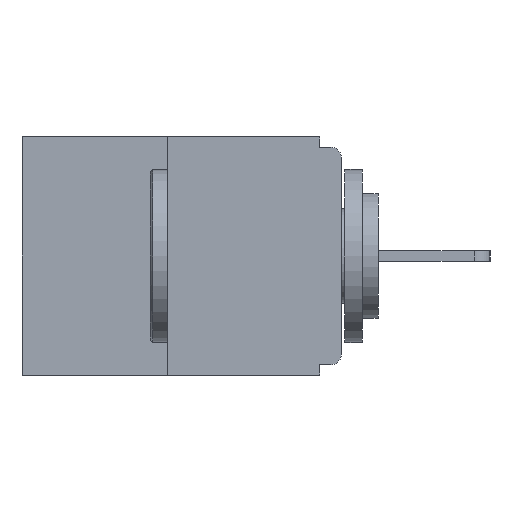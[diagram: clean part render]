
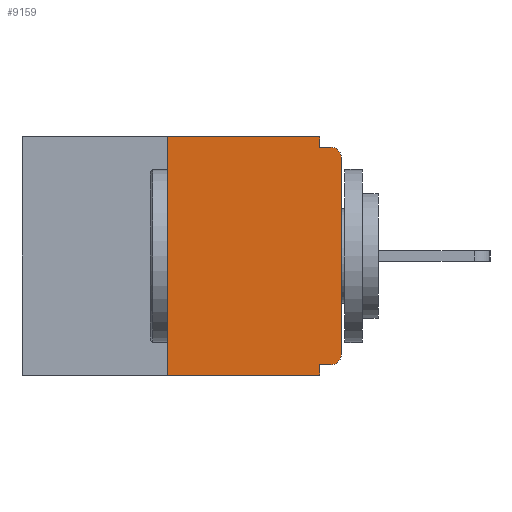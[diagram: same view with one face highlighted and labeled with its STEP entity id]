
A CAD part, left-side view. The second image highlights one B-rep face of the part: STEP entity #9159.
In plain terms, the highlighted planar face has unit normal (-1, 0, 0).
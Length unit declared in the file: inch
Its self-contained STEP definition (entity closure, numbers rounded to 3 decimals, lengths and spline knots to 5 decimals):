
#29 = VERTEX_POINT ( 'NONE', #9714 ) ;
#227 = DIRECTION ( 'NONE',  ( 0., 0., 1. ) ) ;
#543 = DIRECTION ( 'NONE',  ( 0., -1., 0. ) ) ;
#689 = ORIENTED_EDGE ( 'NONE', *, *, #11683, .F. ) ;
#829 = LINE ( 'NONE', #7299, #7676 ) ;
#1295 = VECTOR ( 'NONE', #10471, 39.37008 ) ;
#1308 = DIRECTION ( 'NONE',  ( 0., 0., -1. ) ) ;
#1544 = CARTESIAN_POINT ( 'NONE',  ( 0., 0.015, -0.328 ) ) ;
#1568 = EDGE_CURVE ( 'NONE', #8239, #11762, #11998, .T. ) ;
#1812 = CARTESIAN_POINT ( 'NONE',  ( 0., 0.031, -0.015 ) ) ;
#1931 = ORIENTED_EDGE ( 'NONE', *, *, #9674, .T. ) ;
#1977 = CARTESIAN_POINT ( 'NONE',  ( 0., 0.015, -0.313 ) ) ;
#2024 = DIRECTION ( 'NONE',  ( 0., 0., -1. ) ) ;
#2116 = VERTEX_POINT ( 'NONE', #10322 ) ;
#2307 = VECTOR ( 'NONE', #11942, 39.37008 ) ;
#2414 = DIRECTION ( 'NONE',  ( 1., 0., 0. ) ) ;
#2543 = LINE ( 'NONE', #7018, #12566 ) ;
#2895 = ORIENTED_EDGE ( 'NONE', *, *, #8723, .F. ) ;
#2960 = EDGE_CURVE ( 'NONE', #8239, #29, #11618, .T. ) ;
#3120 = DIRECTION ( 'NONE',  ( 0., 0., -1. ) ) ;
#3128 = CARTESIAN_POINT ( 'NONE',  ( 0., 0.015, -0.03 ) ) ;
#3390 = ORIENTED_EDGE ( 'NONE', *, *, #14428, .F. ) ;
#3425 = VERTEX_POINT ( 'NONE', #1812 ) ;
#3495 = FACE_OUTER_BOUND ( 'NONE', #9658, .T. ) ;
#3520 = EDGE_CURVE ( 'NONE', #29, #8116, #6627, .T. ) ;
#3670 = LINE ( 'NONE', #13601, #4356 ) ;
#3710 = VECTOR ( 'NONE', #4758, 39.37008 ) ;
#3989 = AXIS2_PLACEMENT_3D ( 'NONE', #1977, #8872, #10946 ) ;
#4055 = VERTEX_POINT ( 'NONE', #8600 ) ;
#4114 = CIRCLE ( 'NONE', #10192, 0.015 ) ;
#4356 = VECTOR ( 'NONE', #227, 39.37008 ) ;
#4758 = DIRECTION ( 'NONE',  ( 0., 1., 0. ) ) ;
#4794 = ORIENTED_EDGE ( 'NONE', *, *, #9449, .T. ) ;
#5176 = LINE ( 'NONE', #9640, #2307 ) ;
#5407 = DIRECTION ( 'NONE',  ( -1., 0., 0. ) ) ;
#5536 = DIRECTION ( 'NONE',  ( 0., 0., -1. ) ) ;
#5751 = ORIENTED_EDGE ( 'NONE', *, *, #3520, .F. ) ;
#5980 = AXIS2_PLACEMENT_3D ( 'NONE', #12484, #2414, #1308 ) ;
#6061 = DIRECTION ( 'NONE',  ( 0., 0., 1. ) ) ;
#6122 = ORIENTED_EDGE ( 'NONE', *, *, #1568, .T. ) ;
#6627 = LINE ( 'NONE', #13052, #14257 ) ;
#6967 = CARTESIAN_POINT ( 'NONE',  ( 0., 0., -0.328 ) ) ;
#7018 = CARTESIAN_POINT ( 'NONE',  ( 0., 0., 0. ) ) ;
#7157 = LINE ( 'NONE', #8343, #1295 ) ;
#7299 = CARTESIAN_POINT ( 'NONE',  ( 0., 0.46, 0. ) ) ;
#7344 = ORIENTED_EDGE ( 'NONE', *, *, #2960, .F. ) ;
#7594 = CARTESIAN_POINT ( 'NONE',  ( 0., 0., -0.03 ) ) ;
#7600 = VERTEX_POINT ( 'NONE', #10988 ) ;
#7676 = VECTOR ( 'NONE', #543, 39.37008 ) ;
#7950 = CARTESIAN_POINT ( 'NONE',  ( 0., 0.25, 0. ) ) ;
#7982 = PLANE ( 'NONE',  #5980 ) ;
#8116 = VERTEX_POINT ( 'NONE', #11039 ) ;
#8239 = VERTEX_POINT ( 'NONE', #1544 ) ;
#8248 = ORIENTED_EDGE ( 'NONE', *, *, #9605, .F. ) ;
#8343 = CARTESIAN_POINT ( 'NONE',  ( 0., 0., -0.015 ) ) ;
#8600 = CARTESIAN_POINT ( 'NONE',  ( 0., 0.015, -0.015 ) ) ;
#8723 = EDGE_CURVE ( 'NONE', #2116, #3425, #13407, .T. ) ;
#8747 = VERTEX_POINT ( 'NONE', #7594 ) ;
#8872 = DIRECTION ( 'NONE',  ( -1., 0., 0. ) ) ;
#9159 = ADVANCED_FACE ( 'NONE', ( #3495 ), #7982, .F. ) ;
#9449 = EDGE_CURVE ( 'NONE', #8747, #4055, #4114, .T. ) ;
#9605 = EDGE_CURVE ( 'NONE', #3425, #4055, #7157, .T. ) ;
#9640 = CARTESIAN_POINT ( 'NONE',  ( 0., 0.46, -0.343 ) ) ;
#9658 = EDGE_LOOP ( 'NONE', ( #3390, #689, #10306, #5751, #7344, #6122, #1931, #4794, #8248, #2895 ) ) ;
#9674 = EDGE_CURVE ( 'NONE', #11762, #8747, #2543, .T. ) ;
#9714 = CARTESIAN_POINT ( 'NONE',  ( 0., 0.031, -0.328 ) ) ;
#9905 = VERTEX_POINT ( 'NONE', #7950 ) ;
#10192 = AXIS2_PLACEMENT_3D ( 'NONE', #3128, #5407, #5536 ) ;
#10306 = ORIENTED_EDGE ( 'NONE', *, *, #14494, .T. ) ;
#10322 = CARTESIAN_POINT ( 'NONE',  ( 0., 0.031, 0. ) ) ;
#10471 = DIRECTION ( 'NONE',  ( 0., -1., 0. ) ) ;
#10946 = DIRECTION ( 'NONE',  ( 0., 0., -1. ) ) ;
#10988 = CARTESIAN_POINT ( 'NONE',  ( 0., 0.25, -0.343 ) ) ;
#11039 = CARTESIAN_POINT ( 'NONE',  ( 0., 0.031, -0.343 ) ) ;
#11171 = VECTOR ( 'NONE', #3120, 39.37008 ) ;
#11618 = LINE ( 'NONE', #6967, #3710 ) ;
#11631 = CARTESIAN_POINT ( 'NONE',  ( 0., 0., -0.313 ) ) ;
#11683 = EDGE_CURVE ( 'NONE', #7600, #9905, #3670, .T. ) ;
#11762 = VERTEX_POINT ( 'NONE', #11631 ) ;
#11942 = DIRECTION ( 'NONE',  ( 0., -1., 0. ) ) ;
#11998 = CIRCLE ( 'NONE', #3989, 0.015 ) ;
#12104 = CARTESIAN_POINT ( 'NONE',  ( 0., 0.031, 0. ) ) ;
#12484 = CARTESIAN_POINT ( 'NONE',  ( 0., 0.46, 0. ) ) ;
#12566 = VECTOR ( 'NONE', #6061, 39.37008 ) ;
#13052 = CARTESIAN_POINT ( 'NONE',  ( 0., 0.031, -0.343 ) ) ;
#13407 = LINE ( 'NONE', #12104, #11171 ) ;
#13601 = CARTESIAN_POINT ( 'NONE',  ( 0., 0.25, 0. ) ) ;
#14257 = VECTOR ( 'NONE', #2024, 39.37008 ) ;
#14428 = EDGE_CURVE ( 'NONE', #9905, #2116, #829, .T. ) ;
#14494 = EDGE_CURVE ( 'NONE', #7600, #8116, #5176, .T. ) ;
